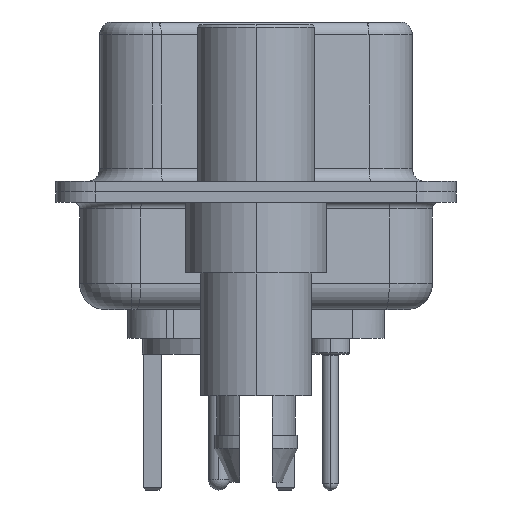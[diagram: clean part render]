
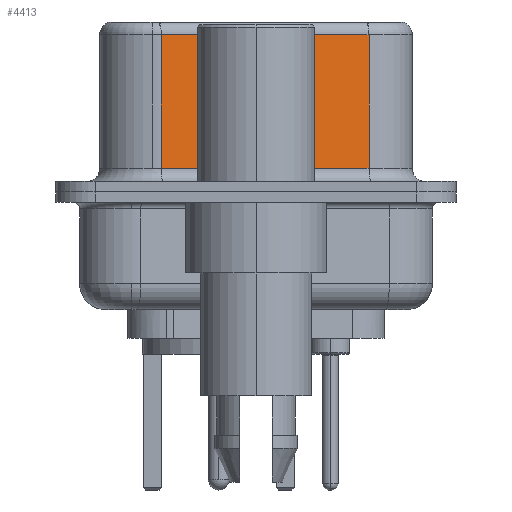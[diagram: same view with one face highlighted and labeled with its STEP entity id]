
A CAD part, left-side view. The second image highlights one B-rep face of the part: STEP entity #4413.
In plain terms, the highlighted planar face has unit normal (-0.985, -0.174, 0).
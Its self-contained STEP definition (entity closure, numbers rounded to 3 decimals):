
#770 = VECTOR ( 'NONE', #19285, 1000. ) ;
#2457 = EDGE_CURVE ( 'NONE', #11286, #16173, #5374, .T. ) ;
#2979 = EDGE_CURVE ( 'NONE', #19216, #11286, #14766, .T. ) ;
#3068 = ORIENTED_EDGE ( 'NONE', *, *, #15671, .T. ) ;
#4413 = ADVANCED_FACE ( 'NONE', ( #21660 ), #22245, .F. ) ;
#4986 = ORIENTED_EDGE ( 'NONE', *, *, #2979, .T. ) ;
#4995 = CARTESIAN_POINT ( 'NONE',  ( 5.132, -4.322, 0.9 ) ) ;
#5251 = ORIENTED_EDGE ( 'NONE', *, *, #22929, .F. ) ;
#5334 = LINE ( 'NONE', #9957, #14758 ) ;
#5374 = LINE ( 'NONE', #4995, #14789 ) ;
#5952 = ORIENTED_EDGE ( 'NONE', *, *, #2457, .T. ) ;
#7845 = DIRECTION ( 'NONE',  ( 0.174, -0.985, 0. ) ) ;
#9957 = CARTESIAN_POINT ( 'NONE',  ( 5.132, -4.322, 6.02 ) ) ;
#11286 = VERTEX_POINT ( 'NONE', #15960 ) ;
#11596 = CARTESIAN_POINT ( 'NONE',  ( 5.132, -4.322, 6.52 ) ) ;
#12153 = AXIS2_PLACEMENT_3D ( 'NONE', #11596, #24125, #23199 ) ;
#13576 = CARTESIAN_POINT ( 'NONE',  ( 5.132, -4.322, 0.9 ) ) ;
#13925 = VERTEX_POINT ( 'NONE', #19691 ) ;
#14758 = VECTOR ( 'NONE', #22960, 1000. ) ;
#14766 = LINE ( 'NONE', #21442, #24005 ) ;
#14789 = VECTOR ( 'NONE', #7845, 1000. ) ;
#15630 = CARTESIAN_POINT ( 'NONE',  ( 5.132, -4.322, 6.52 ) ) ;
#15671 = EDGE_CURVE ( 'NONE', #13925, #19216, #5334, .T. ) ;
#15960 = CARTESIAN_POINT ( 'NONE',  ( 3.73, 3.628, 0.9 ) ) ;
#16173 = VERTEX_POINT ( 'NONE', #13576 ) ;
#19216 = VERTEX_POINT ( 'NONE', #21830 ) ;
#19285 = DIRECTION ( 'NONE',  ( 0., 0., -1. ) ) ;
#19691 = CARTESIAN_POINT ( 'NONE',  ( 5.132, -4.322, 6.02 ) ) ;
#20103 = LINE ( 'NONE', #15630, #770 ) ;
#21442 = CARTESIAN_POINT ( 'NONE',  ( 3.73, 3.628, 6.52 ) ) ;
#21660 = FACE_OUTER_BOUND ( 'NONE', #23419, .T. ) ;
#21830 = CARTESIAN_POINT ( 'NONE',  ( 3.73, 3.628, 6.02 ) ) ;
#22245 = PLANE ( 'NONE',  #12153 ) ;
#22929 = EDGE_CURVE ( 'NONE', #13925, #16173, #20103, .T. ) ;
#22960 = DIRECTION ( 'NONE',  ( -0.174, 0.985, 0. ) ) ;
#23199 = DIRECTION ( 'NONE',  ( -0.174, 0.985, 0. ) ) ;
#23419 = EDGE_LOOP ( 'NONE', ( #5251, #3068, #4986, #5952 ) ) ;
#24005 = VECTOR ( 'NONE', #24198, 1000. ) ;
#24125 = DIRECTION ( 'NONE',  ( 0.985, 0.174, 0. ) ) ;
#24198 = DIRECTION ( 'NONE',  ( 0., 0., -1. ) ) ;
